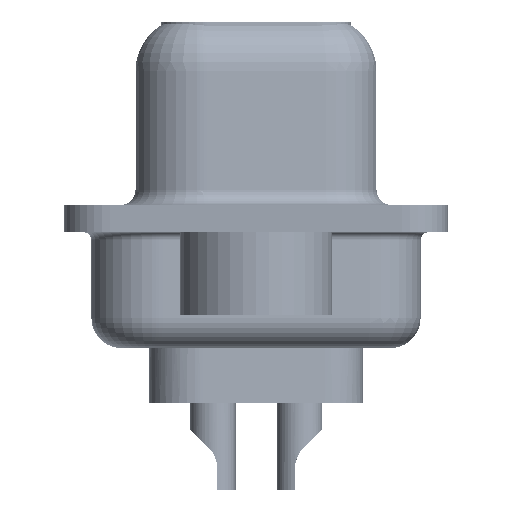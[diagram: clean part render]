
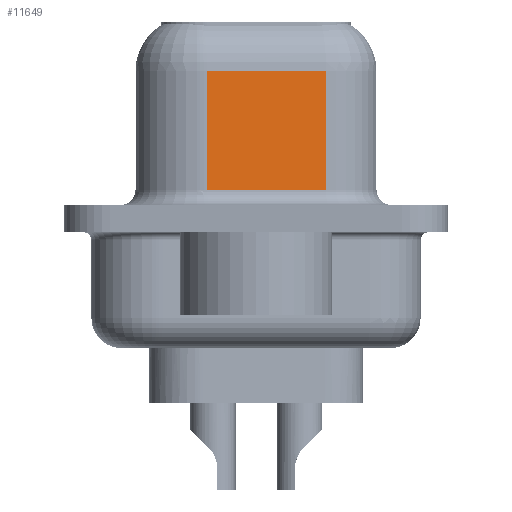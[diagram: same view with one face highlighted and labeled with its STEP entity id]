
A CAD part, left-side view. The second image highlights one B-rep face of the part: STEP entity #11649.
In plain terms, the highlighted planar face has unit normal (-0.985, -0.174, 0).
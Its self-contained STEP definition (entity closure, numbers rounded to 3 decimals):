
#1834 = CARTESIAN_POINT ( 'NONE',  ( 5.068, -2.297, 6.6 ) ) ;
#2936 = CARTESIAN_POINT ( 'NONE',  ( 4.38, 1.603, 0.95 ) ) ;
#3016 = CARTESIAN_POINT ( 'NONE',  ( 5.068, -2.297, 0.95 ) ) ;
#4377 = LINE ( 'NONE', #16959, #21764 ) ;
#4483 = ORIENTED_EDGE ( 'NONE', *, *, #27664, .T. ) ;
#4613 = VECTOR ( 'NONE', #24419, 1000. ) ;
#5100 = DIRECTION ( 'NONE',  ( 0.985, 0.174, 0. ) ) ;
#5523 = ORIENTED_EDGE ( 'NONE', *, *, #25168, .T. ) ;
#5820 = CARTESIAN_POINT ( 'NONE',  ( 5.068, -2.297, 0.95 ) ) ;
#5913 = VERTEX_POINT ( 'NONE', #17431 ) ;
#6256 = CARTESIAN_POINT ( 'NONE',  ( 4.38, 1.603, 6.6 ) ) ;
#10661 = VERTEX_POINT ( 'NONE', #2936 ) ;
#10885 = EDGE_CURVE ( 'NONE', #27669, #18369, #24393, .T. ) ;
#11374 = ORIENTED_EDGE ( 'NONE', *, *, #26219, .T. ) ;
#11395 = LINE ( 'NONE', #6256, #4613 ) ;
#11520 = AXIS2_PLACEMENT_3D ( 'NONE', #20864, #5100, #20964 ) ;
#11649 = ADVANCED_FACE ( 'NONE', ( #13341 ), #16404, .F. ) ;
#12398 = DIRECTION ( 'NONE',  ( -0.174, 0.985, 0. ) ) ;
#13341 = FACE_OUTER_BOUND ( 'NONE', #23237, .T. ) ;
#15449 = DIRECTION ( 'NONE',  ( 0., 0., -1. ) ) ;
#16404 = PLANE ( 'NONE',  #11520 ) ;
#16802 = ORIENTED_EDGE ( 'NONE', *, *, #10885, .F. ) ;
#16959 = CARTESIAN_POINT ( 'NONE',  ( 5.068, -2.297, 4.85 ) ) ;
#17431 = CARTESIAN_POINT ( 'NONE',  ( 4.38, 1.603, 4.85 ) ) ;
#17678 = CARTESIAN_POINT ( 'NONE',  ( 5.068, -2.297, 4.85 ) ) ;
#17830 = LINE ( 'NONE', #5820, #24581 ) ;
#18369 = VERTEX_POINT ( 'NONE', #3016 ) ;
#20864 = CARTESIAN_POINT ( 'NONE',  ( 5.068, -2.297, 6.6 ) ) ;
#20964 = DIRECTION ( 'NONE',  ( -0.174, 0.985, 0. ) ) ;
#21672 = DIRECTION ( 'NONE',  ( 0.174, -0.985, 0. ) ) ;
#21764 = VECTOR ( 'NONE', #12398, 1000. ) ;
#23237 = EDGE_LOOP ( 'NONE', ( #16802, #5523, #4483, #11374 ) ) ;
#23676 = VECTOR ( 'NONE', #15449, 1000. ) ;
#24393 = LINE ( 'NONE', #1834, #23676 ) ;
#24419 = DIRECTION ( 'NONE',  ( 0., 0., -1. ) ) ;
#24581 = VECTOR ( 'NONE', #21672, 1000. ) ;
#25168 = EDGE_CURVE ( 'NONE', #27669, #5913, #4377, .T. ) ;
#26219 = EDGE_CURVE ( 'NONE', #10661, #18369, #17830, .T. ) ;
#27664 = EDGE_CURVE ( 'NONE', #5913, #10661, #11395, .T. ) ;
#27669 = VERTEX_POINT ( 'NONE', #17678 ) ;
